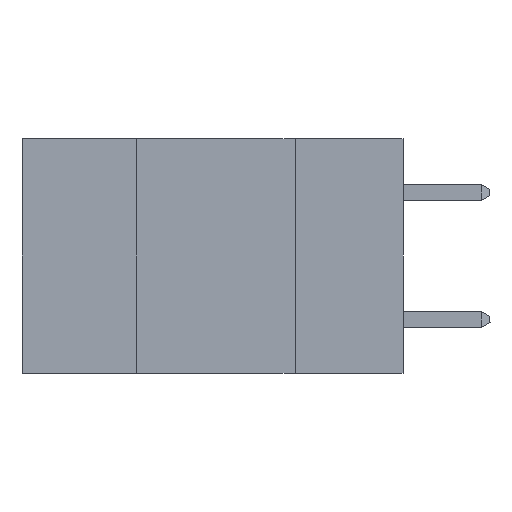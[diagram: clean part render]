
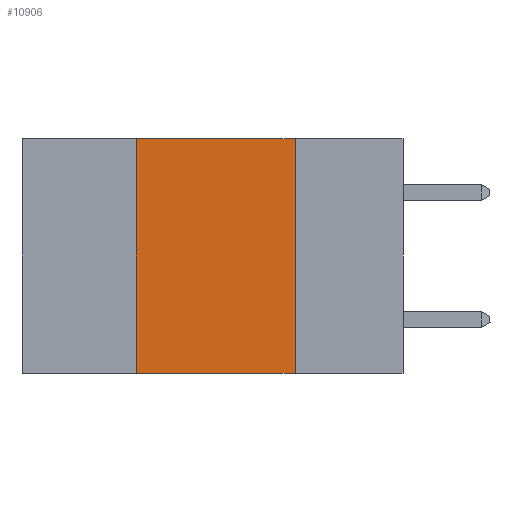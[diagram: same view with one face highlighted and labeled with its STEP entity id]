
A CAD part, left-side view. The second image highlights one B-rep face of the part: STEP entity #10906.
In plain terms, the highlighted planar face has unit normal (-1, 0, 0).
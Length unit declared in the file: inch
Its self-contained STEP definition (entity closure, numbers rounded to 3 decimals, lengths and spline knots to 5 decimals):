
#29 = FACE_OUTER_BOUND ( 'NONE', #6845, .T. ) ;
#2156 = VERTEX_POINT ( 'NONE', #10867 ) ;
#2406 = CARTESIAN_POINT ( 'NONE',  ( 0., 0.42, 0. ) ) ;
#2764 = VECTOR ( 'NONE', #4336, 39.37008 ) ;
#2765 = CARTESIAN_POINT ( 'NONE',  ( 0., 0.6, -0.37 ) ) ;
#2817 = EDGE_CURVE ( 'NONE', #2156, #3823, #2915, .T. ) ;
#2915 = LINE ( 'NONE', #2765, #10990 ) ;
#3068 = DIRECTION ( 'NONE',  ( 0., 0., -1. ) ) ;
#3129 = AXIS2_PLACEMENT_3D ( 'NONE', #9397, #10213, #5361 ) ;
#3396 = VERTEX_POINT ( 'NONE', #3652 ) ;
#3437 = ORIENTED_EDGE ( 'NONE', *, *, #2817, .T. ) ;
#3537 = EDGE_CURVE ( 'NONE', #10678, #3396, #10194, .T. ) ;
#3567 = ORIENTED_EDGE ( 'NONE', *, *, #3537, .F. ) ;
#3652 = CARTESIAN_POINT ( 'NONE',  ( 0., 0.17, 0. ) ) ;
#3722 = ORIENTED_EDGE ( 'NONE', *, *, #4123, .F. ) ;
#3823 = VERTEX_POINT ( 'NONE', #10953 ) ;
#4123 = EDGE_CURVE ( 'NONE', #2156, #10678, #5367, .T. ) ;
#4336 = DIRECTION ( 'NONE',  ( 0., 0., 1. ) ) ;
#4412 = VECTOR ( 'NONE', #6916, 39.37008 ) ;
#4442 = DIRECTION ( 'NONE',  ( 0., -1., 0. ) ) ;
#5279 = CARTESIAN_POINT ( 'NONE',  ( 0., 0.42, 0. ) ) ;
#5361 = DIRECTION ( 'NONE',  ( 0., 0., -1. ) ) ;
#5367 = LINE ( 'NONE', #5279, #2764 ) ;
#6695 = CARTESIAN_POINT ( 'NONE',  ( 0., 0.6, 0. ) ) ;
#6845 = EDGE_LOOP ( 'NONE', ( #7987, #3567, #3722, #3437 ) ) ;
#6916 = DIRECTION ( 'NONE',  ( 0., -1., 0. ) ) ;
#7987 = ORIENTED_EDGE ( 'NONE', *, *, #9837, .F. ) ;
#8496 = VECTOR ( 'NONE', #3068, 39.37008 ) ;
#8554 = PLANE ( 'NONE',  #3129 ) ;
#8899 = CARTESIAN_POINT ( 'NONE',  ( 0., 0.17, 0. ) ) ;
#9397 = CARTESIAN_POINT ( 'NONE',  ( 0., 0.6, 0. ) ) ;
#9837 = EDGE_CURVE ( 'NONE', #3396, #3823, #10683, .T. ) ;
#10194 = LINE ( 'NONE', #6695, #4412 ) ;
#10213 = DIRECTION ( 'NONE',  ( 1., 0., 0. ) ) ;
#10678 = VERTEX_POINT ( 'NONE', #2406 ) ;
#10683 = LINE ( 'NONE', #8899, #8496 ) ;
#10867 = CARTESIAN_POINT ( 'NONE',  ( 0., 0.42, -0.37 ) ) ;
#10906 = ADVANCED_FACE ( 'NONE', ( #29 ), #8554, .F. ) ;
#10953 = CARTESIAN_POINT ( 'NONE',  ( 0., 0.17, -0.37 ) ) ;
#10990 = VECTOR ( 'NONE', #4442, 39.37008 ) ;
